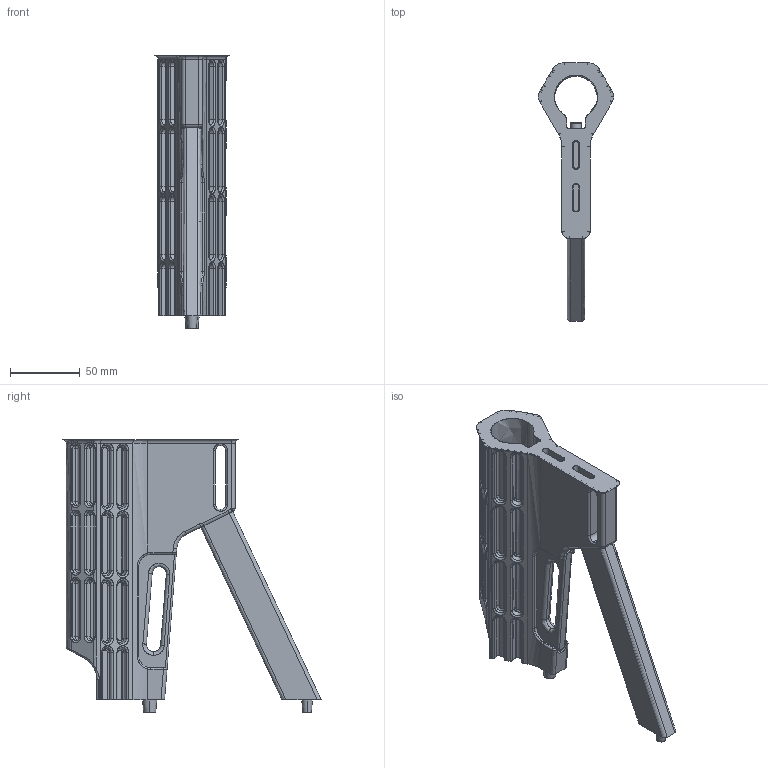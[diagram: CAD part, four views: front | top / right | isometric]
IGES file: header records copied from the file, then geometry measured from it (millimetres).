
Start section: SolidWorks IGES file using analytic representation for surfaces
Global section: file name: Stock body 2.IGS; native system: SolidWorks 2012; preprocessor: SolidWorks 2012; author: Pld; date: 131010.172048; units: inch
Bounding box: 53.81 x 184.75 x 195.11 mm (x, y, z)
Surface area: 96276.3 mm2 (no closed solid volume)
Topology: 0 solids, 0 shells, 673 faces, 6474 edges, 6473 vertices
Faces by surface type: bspline 345, revolution 328
